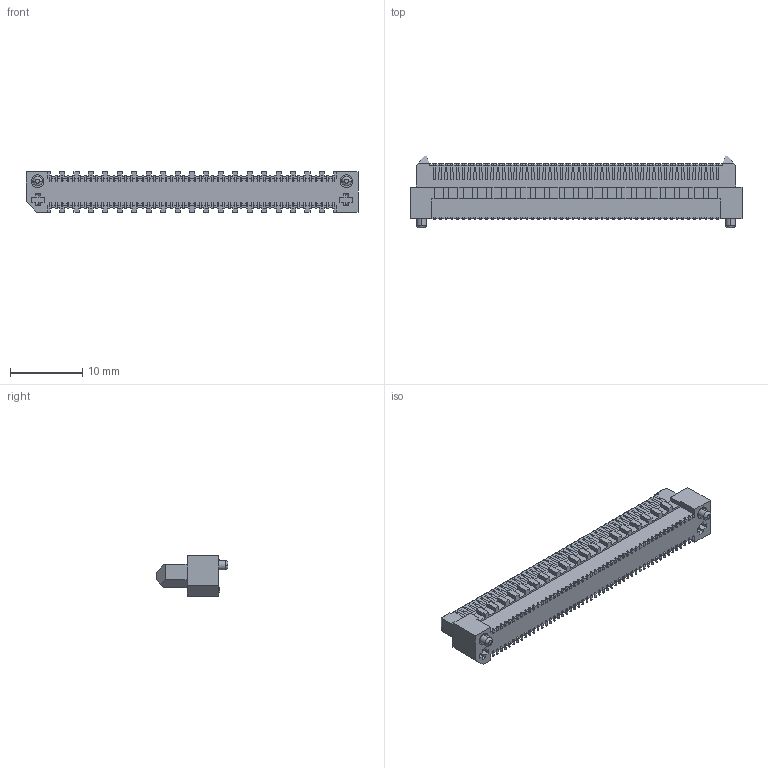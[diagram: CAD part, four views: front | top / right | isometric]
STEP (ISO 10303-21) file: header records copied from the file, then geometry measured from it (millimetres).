
FILE_DESCRIPTION (( 'STEP AP214' ), '1' );
FILE_NAME ('472-100-529-001.STEP', '2020-05-20T13:50:34', ( '' ), ( '' ), 'SwSTEP 2.0', 'SolidWorks 2020', '' );
FILE_SCHEMA (( 'AUTOMOTIVE_DESIGN' ));
Length unit declared in the file: millimetre
Products named in the file (1): 472-100-529-001
Bounding box: 46 x 9.97 x 5.6 mm (x, y, z)
Volume: 1321.4 mm3; surface area: 1437.9 mm2
Topology: 1 solids, 1 shells, 3267 faces, 9348 edges, 6296 vertices
Faces by surface type: plane 2653, cylinder 610, bspline 4
Entity records: 141679 total; most frequent: CARTESIAN_POINT 19656, ORIENTED_EDGE 18696, DIRECTION 16892, EDGE_CURVE 9348, VECTOR 7916, LINE 7916, VERTEX_POINT 6296, AXIS2_PLACEMENT_3D 4488
